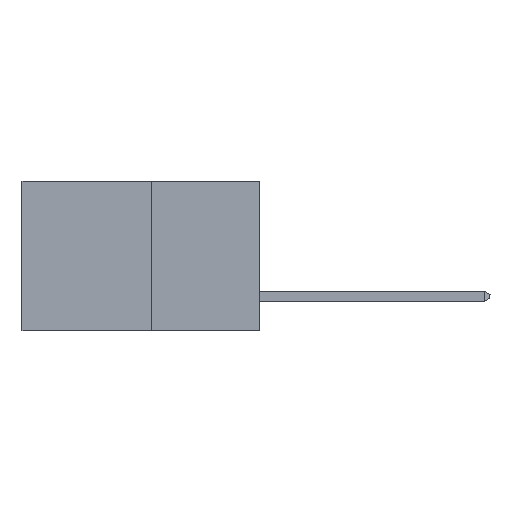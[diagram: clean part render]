
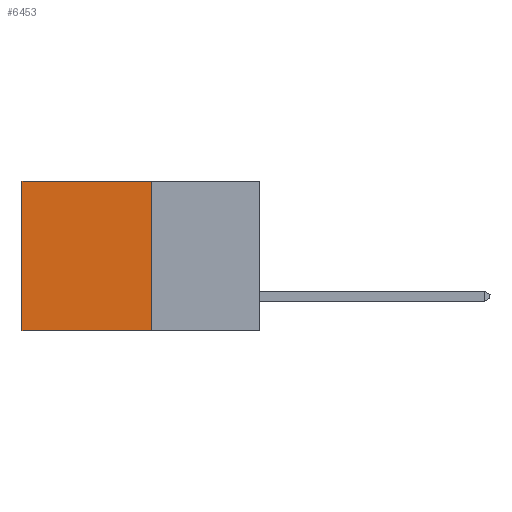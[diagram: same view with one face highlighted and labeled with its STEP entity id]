
A CAD part, left-side view. The second image highlights one B-rep face of the part: STEP entity #6453.
In plain terms, the highlighted planar face has unit normal (-1, 0, 0).
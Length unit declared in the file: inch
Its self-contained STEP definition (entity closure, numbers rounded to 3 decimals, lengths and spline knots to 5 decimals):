
#770 = EDGE_CURVE ( 'NONE', #7622, #5491, #12608, .T. ) ;
#2662 = CARTESIAN_POINT ( 'NONE',  ( 0.277, 0.59, -0.37 ) ) ;
#3447 = CARTESIAN_POINT ( 'NONE',  ( 0.277, 0.27, 0. ) ) ;
#4184 = DIRECTION ( 'NONE',  ( 1., 0., 0. ) ) ;
#5294 = LINE ( 'NONE', #14566, #27610 ) ;
#5491 = VERTEX_POINT ( 'NONE', #9470 ) ;
#6453 = ADVANCED_FACE ( 'NONE', ( #11496 ), #14156, .F. ) ;
#6554 = VECTOR ( 'NONE', #25204, 39.37008 ) ;
#6697 = VECTOR ( 'NONE', #16745, 39.37008 ) ;
#7622 = VERTEX_POINT ( 'NONE', #3447 ) ;
#8620 = VECTOR ( 'NONE', #21673, 39.37008 ) ;
#9470 = CARTESIAN_POINT ( 'NONE',  ( 0.277, 0.59, 0. ) ) ;
#11496 = FACE_OUTER_BOUND ( 'NONE', #31355, .T. ) ;
#12608 = LINE ( 'NONE', #29157, #6697 ) ;
#13220 = LINE ( 'NONE', #29923, #6554 ) ;
#14156 = PLANE ( 'NONE',  #17974 ) ;
#14333 = CARTESIAN_POINT ( 'NONE',  ( 0.277, 0.27, -0.37 ) ) ;
#14566 = CARTESIAN_POINT ( 'NONE',  ( 0.277, 0.27, -0.37 ) ) ;
#14583 = EDGE_CURVE ( 'NONE', #14679, #20488, #27427, .T. ) ;
#14679 = VERTEX_POINT ( 'NONE', #19541 ) ;
#15524 = ORIENTED_EDGE ( 'NONE', *, *, #14583, .F. ) ;
#16745 = DIRECTION ( 'NONE',  ( 0., 1., 0. ) ) ;
#17974 = AXIS2_PLACEMENT_3D ( 'NONE', #19065, #4184, #21502 ) ;
#19065 = CARTESIAN_POINT ( 'NONE',  ( 0.277, 0.27, -0.37 ) ) ;
#19410 = ORIENTED_EDGE ( 'NONE', *, *, #770, .T. ) ;
#19541 = CARTESIAN_POINT ( 'NONE',  ( 0.277, 0.27, -0.37 ) ) ;
#19560 = EDGE_CURVE ( 'NONE', #7622, #14679, #5294, .T. ) ;
#20488 = VERTEX_POINT ( 'NONE', #2662 ) ;
#21502 = DIRECTION ( 'NONE',  ( 0., 0., -1. ) ) ;
#21673 = DIRECTION ( 'NONE',  ( 0., 1., 0. ) ) ;
#23021 = ORIENTED_EDGE ( 'NONE', *, *, #27038, .T. ) ;
#25204 = DIRECTION ( 'NONE',  ( 0., 0., -1. ) ) ;
#27038 = EDGE_CURVE ( 'NONE', #5491, #20488, #13220, .T. ) ;
#27427 = LINE ( 'NONE', #14333, #8620 ) ;
#27610 = VECTOR ( 'NONE', #31449, 39.37008 ) ;
#28643 = ORIENTED_EDGE ( 'NONE', *, *, #19560, .F. ) ;
#29157 = CARTESIAN_POINT ( 'NONE',  ( 0.277, 0.27, 0. ) ) ;
#29923 = CARTESIAN_POINT ( 'NONE',  ( 0.277, 0.59, -0.37 ) ) ;
#31355 = EDGE_LOOP ( 'NONE', ( #23021, #15524, #28643, #19410 ) ) ;
#31449 = DIRECTION ( 'NONE',  ( 0., 0., -1. ) ) ;
